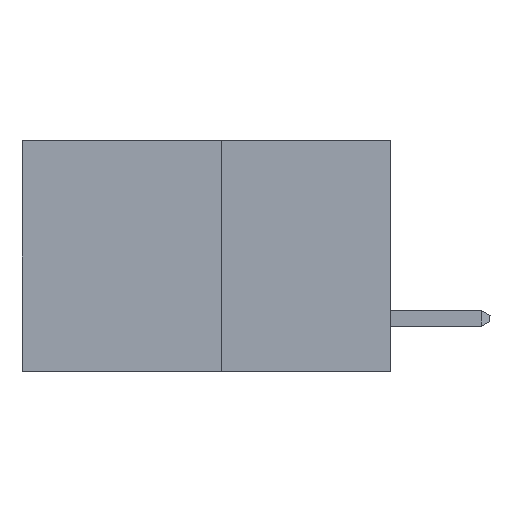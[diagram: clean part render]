
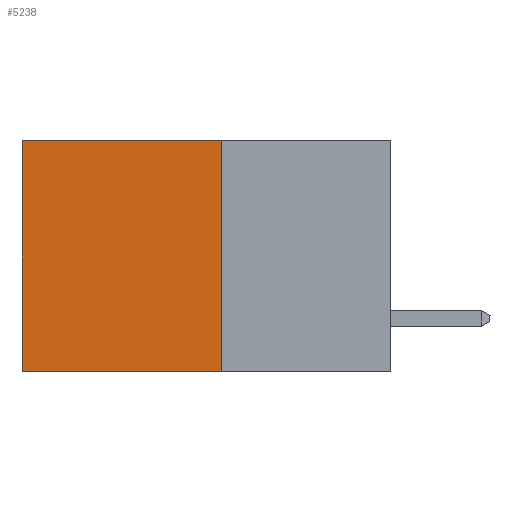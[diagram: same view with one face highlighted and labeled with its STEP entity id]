
A CAD part, left-side view. The second image highlights one B-rep face of the part: STEP entity #5238.
In plain terms, the highlighted planar face has unit normal (-1, 0, 0).
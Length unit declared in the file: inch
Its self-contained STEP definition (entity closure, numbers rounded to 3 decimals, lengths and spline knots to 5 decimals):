
#1351 = LINE ( 'NONE', #9832, #4710 ) ;
#2171 = LINE ( 'NONE', #17803, #14944 ) ;
#2920 = VERTEX_POINT ( 'NONE', #10545 ) ;
#3011 = EDGE_CURVE ( 'NONE', #13082, #16075, #1351, .T. ) ;
#4395 = ORIENTED_EDGE ( 'NONE', *, *, #16179, .F. ) ;
#4710 = VECTOR ( 'NONE', #9958, 39.37008 ) ;
#5238 = ADVANCED_FACE ( 'NONE', ( #10623 ), #14692, .F. ) ;
#5511 = CARTESIAN_POINT ( 'NONE',  ( 0.277, 0.27, -0.37 ) ) ;
#5530 = DIRECTION ( 'NONE',  ( 0., 1., 0. ) ) ;
#5864 = CARTESIAN_POINT ( 'NONE',  ( 0.277, 0.27, 0. ) ) ;
#6017 = EDGE_CURVE ( 'NONE', #8575, #2920, #8254, .T. ) ;
#6771 = AXIS2_PLACEMENT_3D ( 'NONE', #14529, #14507, #14488 ) ;
#8254 = LINE ( 'NONE', #5511, #12678 ) ;
#8575 = VERTEX_POINT ( 'NONE', #14963 ) ;
#9229 = EDGE_LOOP ( 'NONE', ( #10293, #9330, #4395, #18612 ) ) ;
#9290 = LINE ( 'NONE', #18763, #17587 ) ;
#9330 = ORIENTED_EDGE ( 'NONE', *, *, #6017, .F. ) ;
#9538 = DIRECTION ( 'NONE',  ( 0., 0., -1. ) ) ;
#9832 = CARTESIAN_POINT ( 'NONE',  ( 0.277, 0.27, 0. ) ) ;
#9958 = DIRECTION ( 'NONE',  ( 0., 1., 0. ) ) ;
#10293 = ORIENTED_EDGE ( 'NONE', *, *, #11889, .T. ) ;
#10545 = CARTESIAN_POINT ( 'NONE',  ( 0.277, 0.59, -0.37 ) ) ;
#10623 = FACE_OUTER_BOUND ( 'NONE', #9229, .T. ) ;
#11889 = EDGE_CURVE ( 'NONE', #16075, #2920, #2171, .T. ) ;
#11999 = CARTESIAN_POINT ( 'NONE',  ( 0.277, 0.59, 0. ) ) ;
#12678 = VECTOR ( 'NONE', #5530, 39.37008 ) ;
#13082 = VERTEX_POINT ( 'NONE', #5864 ) ;
#13942 = DIRECTION ( 'NONE',  ( 0., 0., -1. ) ) ;
#14488 = DIRECTION ( 'NONE',  ( 0., 0., -1. ) ) ;
#14507 = DIRECTION ( 'NONE',  ( 1., 0., 0. ) ) ;
#14529 = CARTESIAN_POINT ( 'NONE',  ( 0.277, 0.27, -0.37 ) ) ;
#14692 = PLANE ( 'NONE',  #6771 ) ;
#14944 = VECTOR ( 'NONE', #9538, 39.37008 ) ;
#14963 = CARTESIAN_POINT ( 'NONE',  ( 0.277, 0.27, -0.37 ) ) ;
#16075 = VERTEX_POINT ( 'NONE', #11999 ) ;
#16179 = EDGE_CURVE ( 'NONE', #13082, #8575, #9290, .T. ) ;
#17587 = VECTOR ( 'NONE', #13942, 39.37008 ) ;
#17803 = CARTESIAN_POINT ( 'NONE',  ( 0.277, 0.59, -0.37 ) ) ;
#18612 = ORIENTED_EDGE ( 'NONE', *, *, #3011, .T. ) ;
#18763 = CARTESIAN_POINT ( 'NONE',  ( 0.277, 0.27, -0.37 ) ) ;
